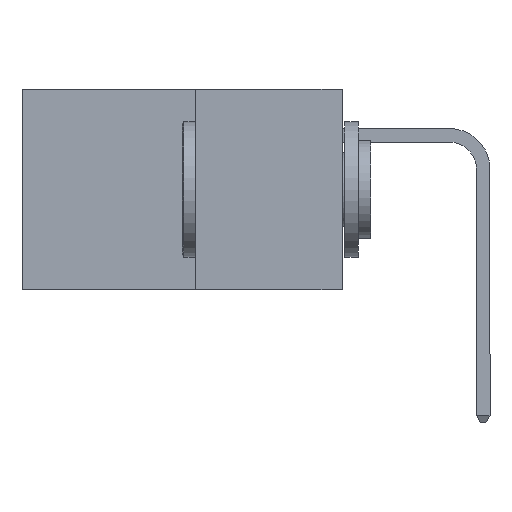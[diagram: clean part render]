
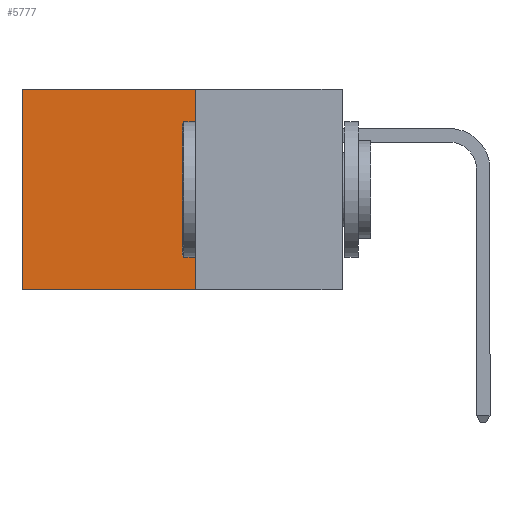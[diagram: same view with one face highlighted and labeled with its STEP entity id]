
A CAD part, left-side view. The second image highlights one B-rep face of the part: STEP entity #5777.
In plain terms, the highlighted planar face has unit normal (-1, 0, 0).
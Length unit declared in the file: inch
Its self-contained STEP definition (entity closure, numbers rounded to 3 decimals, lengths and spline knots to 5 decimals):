
#324 = VERTEX_POINT ( 'NONE', #5496 ) ;
#521 = EDGE_CURVE ( 'NONE', #4136, #6435, #7279, .T. ) ;
#684 = ORIENTED_EDGE ( 'NONE', *, *, #2009, .T. ) ;
#836 = CARTESIAN_POINT ( 'NONE',  ( 0.277, 0.27, 0. ) ) ;
#1181 = ORIENTED_EDGE ( 'NONE', *, *, #5397, .F. ) ;
#1215 = CARTESIAN_POINT ( 'NONE',  ( 0.277, 0.27, -0.37 ) ) ;
#1346 = DIRECTION ( 'NONE',  ( 0., 0., -1. ) ) ;
#1401 = ORIENTED_EDGE ( 'NONE', *, *, #521, .T. ) ;
#2009 = EDGE_CURVE ( 'NONE', #6435, #324, #4651, .T. ) ;
#3430 = EDGE_LOOP ( 'NONE', ( #684, #6570, #1181, #1401 ) ) ;
#3924 = VECTOR ( 'NONE', #9352, 39.37008 ) ;
#4136 = VERTEX_POINT ( 'NONE', #836 ) ;
#4137 = CARTESIAN_POINT ( 'NONE',  ( 0.277, 0.59, -0.37 ) ) ;
#4366 = DIRECTION ( 'NONE',  ( 0., 1., 0. ) ) ;
#4414 = VECTOR ( 'NONE', #9131, 39.37008 ) ;
#4625 = VECTOR ( 'NONE', #1346, 39.37008 ) ;
#4651 = LINE ( 'NONE', #4137, #4414 ) ;
#4867 = LINE ( 'NONE', #1215, #4625 ) ;
#4883 = CARTESIAN_POINT ( 'NONE',  ( 0.277, 0.59, 0. ) ) ;
#5209 = CARTESIAN_POINT ( 'NONE',  ( 0.277, 0.27, -0.37 ) ) ;
#5366 = VECTOR ( 'NONE', #4366, 39.37008 ) ;
#5397 = EDGE_CURVE ( 'NONE', #4136, #8067, #4867, .T. ) ;
#5491 = EDGE_CURVE ( 'NONE', #8067, #324, #7778, .T. ) ;
#5496 = CARTESIAN_POINT ( 'NONE',  ( 0.277, 0.59, -0.37 ) ) ;
#5777 = ADVANCED_FACE ( 'NONE', ( #5985 ), #8170, .F. ) ;
#5985 = FACE_OUTER_BOUND ( 'NONE', #3430, .T. ) ;
#6435 = VERTEX_POINT ( 'NONE', #4883 ) ;
#6570 = ORIENTED_EDGE ( 'NONE', *, *, #5491, .F. ) ;
#6578 = CARTESIAN_POINT ( 'NONE',  ( 0.277, 0.27, 0. ) ) ;
#7279 = LINE ( 'NONE', #6578, #5366 ) ;
#7778 = LINE ( 'NONE', #9343, #3924 ) ;
#8056 = DIRECTION ( 'NONE',  ( 0., 0., -1. ) ) ;
#8067 = VERTEX_POINT ( 'NONE', #5209 ) ;
#8073 = DIRECTION ( 'NONE',  ( 1., 0., 0. ) ) ;
#8123 = CARTESIAN_POINT ( 'NONE',  ( 0.277, 0.27, -0.37 ) ) ;
#8170 = PLANE ( 'NONE',  #9087 ) ;
#9087 = AXIS2_PLACEMENT_3D ( 'NONE', #8123, #8073, #8056 ) ;
#9131 = DIRECTION ( 'NONE',  ( 0., 0., -1. ) ) ;
#9343 = CARTESIAN_POINT ( 'NONE',  ( 0.277, 0.27, -0.37 ) ) ;
#9352 = DIRECTION ( 'NONE',  ( 0., 1., 0. ) ) ;
